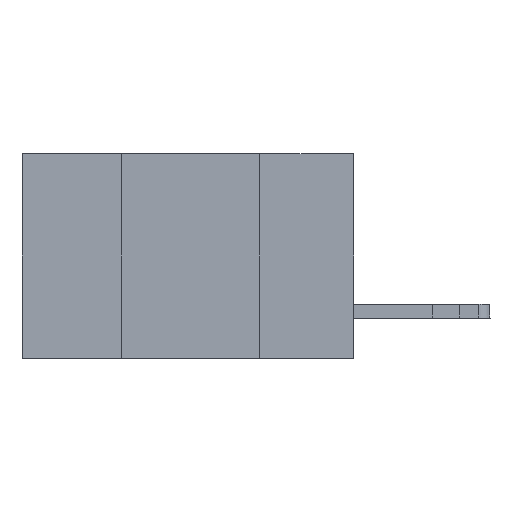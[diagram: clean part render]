
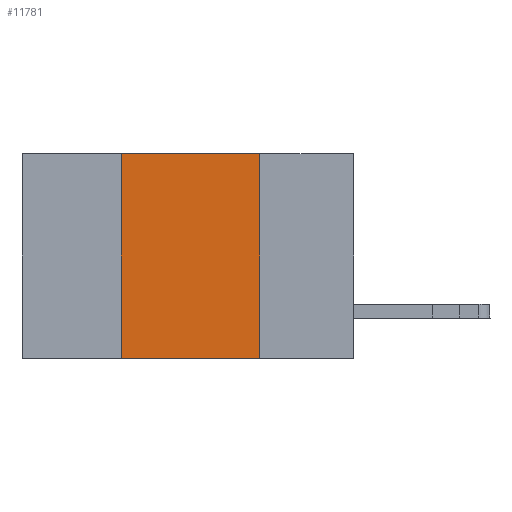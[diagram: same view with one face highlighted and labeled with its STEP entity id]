
A CAD part, left-side view. The second image highlights one B-rep face of the part: STEP entity #11781.
In plain terms, the highlighted planar face has unit normal (-1, 0, 0).
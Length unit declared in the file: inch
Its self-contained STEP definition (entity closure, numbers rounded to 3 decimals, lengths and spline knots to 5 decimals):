
#353 = VERTEX_POINT ( 'NONE', #15883 ) ;
#681 = CARTESIAN_POINT ( 'NONE',  ( 0., 0.6, 0. ) ) ;
#2193 = CARTESIAN_POINT ( 'NONE',  ( 0., 0.6, -0.37 ) ) ;
#3603 = DIRECTION ( 'NONE',  ( 0., 0., -1. ) ) ;
#4345 = VECTOR ( 'NONE', #17336, 39.37008 ) ;
#5411 = AXIS2_PLACEMENT_3D ( 'NONE', #681, #28712, #13588 ) ;
#5524 = VECTOR ( 'NONE', #9854, 39.37008 ) ;
#5943 = EDGE_CURVE ( 'NONE', #26742, #353, #19847, .T. ) ;
#6349 = VERTEX_POINT ( 'NONE', #29208 ) ;
#6542 = FACE_OUTER_BOUND ( 'NONE', #31977, .T. ) ;
#8763 = VECTOR ( 'NONE', #10275, 39.37008 ) ;
#9854 = DIRECTION ( 'NONE',  ( 0., -1., 0. ) ) ;
#9969 = CARTESIAN_POINT ( 'NONE',  ( 0., 0.42, -0.37 ) ) ;
#10275 = DIRECTION ( 'NONE',  ( 0., 0., 1. ) ) ;
#11781 = ADVANCED_FACE ( 'NONE', ( #6542 ), #23705, .F. ) ;
#11783 = LINE ( 'NONE', #31356, #16939 ) ;
#12740 = CARTESIAN_POINT ( 'NONE',  ( 0., 0.42, 0. ) ) ;
#13547 = ORIENTED_EDGE ( 'NONE', *, *, #29006, .F. ) ;
#13588 = DIRECTION ( 'NONE',  ( 0., 0., -1. ) ) ;
#14198 = ORIENTED_EDGE ( 'NONE', *, *, #30667, .F. ) ;
#14627 = ORIENTED_EDGE ( 'NONE', *, *, #20562, .T. ) ;
#14991 = CARTESIAN_POINT ( 'NONE',  ( 0., 0.6, 0. ) ) ;
#15883 = CARTESIAN_POINT ( 'NONE',  ( 0., 0.17, 0. ) ) ;
#16349 = LINE ( 'NONE', #22975, #8763 ) ;
#16886 = ORIENTED_EDGE ( 'NONE', *, *, #5943, .F. ) ;
#16939 = VECTOR ( 'NONE', #3603, 39.37008 ) ;
#17336 = DIRECTION ( 'NONE',  ( 0., -1., 0. ) ) ;
#19847 = LINE ( 'NONE', #14991, #5524 ) ;
#20562 = EDGE_CURVE ( 'NONE', #27971, #6349, #24638, .T. ) ;
#22975 = CARTESIAN_POINT ( 'NONE',  ( 0., 0.42, 0. ) ) ;
#23705 = PLANE ( 'NONE',  #5411 ) ;
#24638 = LINE ( 'NONE', #2193, #4345 ) ;
#26742 = VERTEX_POINT ( 'NONE', #12740 ) ;
#27971 = VERTEX_POINT ( 'NONE', #9969 ) ;
#28712 = DIRECTION ( 'NONE',  ( 1., 0., 0. ) ) ;
#29006 = EDGE_CURVE ( 'NONE', #353, #6349, #11783, .T. ) ;
#29208 = CARTESIAN_POINT ( 'NONE',  ( 0., 0.17, -0.37 ) ) ;
#30667 = EDGE_CURVE ( 'NONE', #27971, #26742, #16349, .T. ) ;
#31356 = CARTESIAN_POINT ( 'NONE',  ( 0., 0.17, 0. ) ) ;
#31977 = EDGE_LOOP ( 'NONE', ( #13547, #16886, #14198, #14627 ) ) ;
